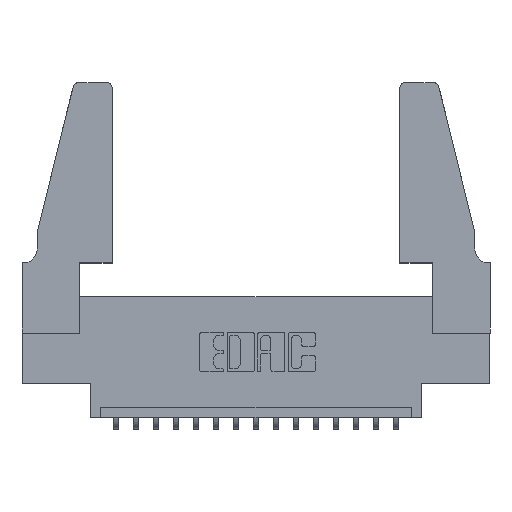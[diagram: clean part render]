
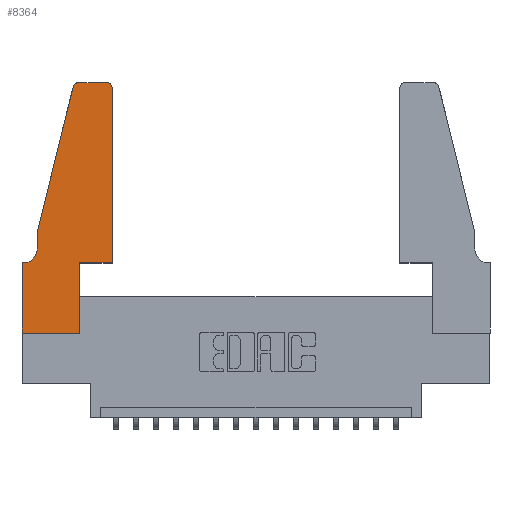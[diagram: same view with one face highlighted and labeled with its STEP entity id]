
A CAD part, top view. The second image highlights one B-rep face of the part: STEP entity #8364.
In plain terms, the highlighted planar face has unit normal (0, 0, 1).
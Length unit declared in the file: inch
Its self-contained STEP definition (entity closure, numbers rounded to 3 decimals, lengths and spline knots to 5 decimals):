
#66 = CARTESIAN_POINT ( 'NONE',  ( 0., 0., 0.37 ) ) ;
#168 = VERTEX_POINT ( 'NONE', #4830 ) ;
#230 = ORIENTED_EDGE ( 'NONE', *, *, #2581, .T. ) ;
#423 = CARTESIAN_POINT ( 'NONE',  ( 0.4205, 1.22, 0.37 ) ) ;
#506 = LINE ( 'NONE', #14477, #10344 ) ;
#517 = VERTEX_POINT ( 'NONE', #4831 ) ;
#727 = ORIENTED_EDGE ( 'NONE', *, *, #1288, .T. ) ;
#811 = CARTESIAN_POINT ( 'NONE',  ( 0.4505, 0.35, 0.37 ) ) ;
#1288 = EDGE_CURVE ( 'NONE', #4576, #8995, #12012, .T. ) ;
#1664 = VECTOR ( 'NONE', #2609, 39.37008 ) ;
#1736 = VERTEX_POINT ( 'NONE', #11923 ) ;
#1748 = EDGE_CURVE ( 'NONE', #517, #8963, #506, .T. ) ;
#1861 = AXIS2_PLACEMENT_3D ( 'NONE', #3025, #12370, #14889 ) ;
#2049 = EDGE_CURVE ( 'NONE', #8366, #517, #5512, .T. ) ;
#2075 = CARTESIAN_POINT ( 'NONE',  ( 0.0755, 0.42, 0.37 ) ) ;
#2421 = EDGE_CURVE ( 'NONE', #168, #3109, #10129, .T. ) ;
#2470 = VERTEX_POINT ( 'NONE', #13424 ) ;
#2581 = EDGE_CURVE ( 'NONE', #8963, #15738, #5514, .T. ) ;
#2609 = DIRECTION ( 'NONE',  ( 0., 1., 0. ) ) ;
#2863 = CARTESIAN_POINT ( 'NONE',  ( 0., 0.35, 0.37 ) ) ;
#2999 = ORIENTED_EDGE ( 'NONE', *, *, #2049, .T. ) ;
#3025 = CARTESIAN_POINT ( 'NONE',  ( 0.284, 1.22, 0.37 ) ) ;
#3109 = VERTEX_POINT ( 'NONE', #8748 ) ;
#3320 = AXIS2_PLACEMENT_3D ( 'NONE', #423, #9788, #6195 ) ;
#3775 = VERTEX_POINT ( 'NONE', #12966 ) ;
#3779 = DIRECTION ( 'NONE',  ( -1., 0., 0. ) ) ;
#4156 = CARTESIAN_POINT ( 'NONE',  ( 0.4505, 1.22, 0.37 ) ) ;
#4158 = CARTESIAN_POINT ( 'NONE',  ( 0.0055, 0.35, 0.37 ) ) ;
#4191 = DIRECTION ( 'NONE',  ( 1., 0., 0. ) ) ;
#4576 = VERTEX_POINT ( 'NONE', #2075 ) ;
#4629 = ORIENTED_EDGE ( 'NONE', *, *, #10245, .T. ) ;
#4635 = AXIS2_PLACEMENT_3D ( 'NONE', #6333, #6272, #3779 ) ;
#4735 = EDGE_CURVE ( 'NONE', #3775, #9260, #9199, .T. ) ;
#4830 = CARTESIAN_POINT ( 'NONE',  ( 0., 0.35, 0.37 ) ) ;
#4831 = CARTESIAN_POINT ( 'NONE',  ( 0.4205, 1.25, 0.37 ) ) ;
#4851 = EDGE_CURVE ( 'NONE', #1736, #3775, #5220, .T. ) ;
#5013 = CARTESIAN_POINT ( 'NONE',  ( 0.4505, 0.35, 0.37 ) ) ;
#5220 = LINE ( 'NONE', #14694, #1664 ) ;
#5512 = CIRCLE ( 'NONE', #3320, 0.03 ) ;
#5514 = CIRCLE ( 'NONE', #1861, 0.03 ) ;
#5660 = DIRECTION ( 'NONE',  ( -0.239, -0.971, 0. ) ) ;
#6049 = EDGE_CURVE ( 'NONE', #9260, #8366, #9267, .T. ) ;
#6173 = EDGE_CURVE ( 'NONE', #15738, #2470, #16560, .T. ) ;
#6195 = DIRECTION ( 'NONE',  ( 1., 0., 0. ) ) ;
#6272 = DIRECTION ( 'NONE',  ( 0., 0., -1. ) ) ;
#6333 = CARTESIAN_POINT ( 'NONE',  ( 0.0055, 0.42, 0.37 ) ) ;
#6467 = VECTOR ( 'NONE', #16492, 39.37008 ) ;
#6726 = CARTESIAN_POINT ( 'NONE',  ( 0.284, 1.25, 0.37 ) ) ;
#7290 = EDGE_CURVE ( 'NONE', #2470, #4576, #12735, .T. ) ;
#7314 = EDGE_LOOP ( 'NONE', ( #11023, #230, #12596, #16667, #727, #4629, #7611, #12759, #16702, #8628, #10194, #2999 ) ) ;
#7611 = ORIENTED_EDGE ( 'NONE', *, *, #2421, .T. ) ;
#7661 = DIRECTION ( 'NONE',  ( -1., 0., 0. ) ) ;
#8126 = PLANE ( 'NONE',  #16028 ) ;
#8364 = ADVANCED_FACE ( 'NONE', ( #16474 ), #8126, .T. ) ;
#8366 = VERTEX_POINT ( 'NONE', #4156 ) ;
#8387 = LINE ( 'NONE', #10970, #13595 ) ;
#8628 = ORIENTED_EDGE ( 'NONE', *, *, #4735, .T. ) ;
#8748 = CARTESIAN_POINT ( 'NONE',  ( 0., 0., 0.37 ) ) ;
#8963 = VERTEX_POINT ( 'NONE', #6726 ) ;
#8995 = VERTEX_POINT ( 'NONE', #4158 ) ;
#9139 = LINE ( 'NONE', #9982, #10186 ) ;
#9199 = LINE ( 'NONE', #5013, #9829 ) ;
#9260 = VERTEX_POINT ( 'NONE', #811 ) ;
#9267 = LINE ( 'NONE', #15028, #14892 ) ;
#9495 = DIRECTION ( 'NONE',  ( 1., 0., 0. ) ) ;
#9512 = CARTESIAN_POINT ( 'NONE',  ( 0.25487, 1.22718, 0.37 ) ) ;
#9788 = DIRECTION ( 'NONE',  ( 0., 0., 1. ) ) ;
#9801 = CARTESIAN_POINT ( 'NONE',  ( 0.0755, 0.5, 0.37 ) ) ;
#9829 = VECTOR ( 'NONE', #11835, 39.37008 ) ;
#9982 = CARTESIAN_POINT ( 'NONE',  ( 0.0755, 0.35, 0.37 ) ) ;
#10129 = LINE ( 'NONE', #66, #10531 ) ;
#10186 = VECTOR ( 'NONE', #16619, 39.37008 ) ;
#10194 = ORIENTED_EDGE ( 'NONE', *, *, #6049, .T. ) ;
#10245 = EDGE_CURVE ( 'NONE', #8995, #168, #9139, .T. ) ;
#10344 = VECTOR ( 'NONE', #7661, 39.37008 ) ;
#10531 = VECTOR ( 'NONE', #12030, 39.37008 ) ;
#10970 = CARTESIAN_POINT ( 'NONE',  ( 0., 0., 0.37 ) ) ;
#11023 = ORIENTED_EDGE ( 'NONE', *, *, #1748, .T. ) ;
#11835 = DIRECTION ( 'NONE',  ( 1., 0., 0. ) ) ;
#11923 = CARTESIAN_POINT ( 'NONE',  ( 0.2865, 0., 0.37 ) ) ;
#12012 = CIRCLE ( 'NONE', #4635, 0.07 ) ;
#12030 = DIRECTION ( 'NONE',  ( 0., -1., 0. ) ) ;
#12370 = DIRECTION ( 'NONE',  ( 0., 0., 1. ) ) ;
#12596 = ORIENTED_EDGE ( 'NONE', *, *, #6173, .T. ) ;
#12735 = LINE ( 'NONE', #9801, #6467 ) ;
#12759 = ORIENTED_EDGE ( 'NONE', *, *, #13933, .T. ) ;
#12966 = CARTESIAN_POINT ( 'NONE',  ( 0.2865, 0.35, 0.37 ) ) ;
#13424 = CARTESIAN_POINT ( 'NONE',  ( 0.0755, 0.5, 0.37 ) ) ;
#13594 = CARTESIAN_POINT ( 'NONE',  ( 0.0755, 0.5, 0.37 ) ) ;
#13595 = VECTOR ( 'NONE', #4191, 39.37008 ) ;
#13933 = EDGE_CURVE ( 'NONE', #3109, #1736, #8387, .T. ) ;
#14477 = CARTESIAN_POINT ( 'NONE',  ( 0.2605, 1.25, 0.37 ) ) ;
#14654 = DIRECTION ( 'NONE',  ( 0., 0., 1. ) ) ;
#14694 = CARTESIAN_POINT ( 'NONE',  ( 0.2865, 0.35, 0.37 ) ) ;
#14889 = DIRECTION ( 'NONE',  ( 1., 0., 0. ) ) ;
#14892 = VECTOR ( 'NONE', #16373, 39.37008 ) ;
#15028 = CARTESIAN_POINT ( 'NONE',  ( 0.4505, 0.35, 0.37 ) ) ;
#15738 = VERTEX_POINT ( 'NONE', #9512 ) ;
#16028 = AXIS2_PLACEMENT_3D ( 'NONE', #2863, #14654, #9495 ) ;
#16373 = DIRECTION ( 'NONE',  ( 0., 1., 0. ) ) ;
#16474 = FACE_OUTER_BOUND ( 'NONE', #7314, .T. ) ;
#16492 = DIRECTION ( 'NONE',  ( 0., -1., 0. ) ) ;
#16560 = LINE ( 'NONE', #13594, #16971 ) ;
#16619 = DIRECTION ( 'NONE',  ( -1., 0., 0. ) ) ;
#16667 = ORIENTED_EDGE ( 'NONE', *, *, #7290, .T. ) ;
#16702 = ORIENTED_EDGE ( 'NONE', *, *, #4851, .T. ) ;
#16971 = VECTOR ( 'NONE', #5660, 39.37008 ) ;
